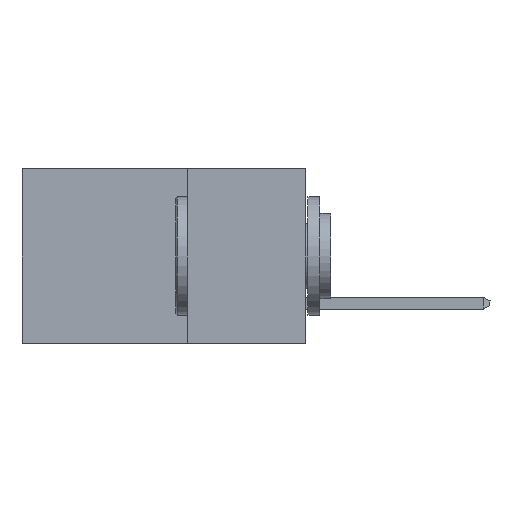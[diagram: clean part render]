
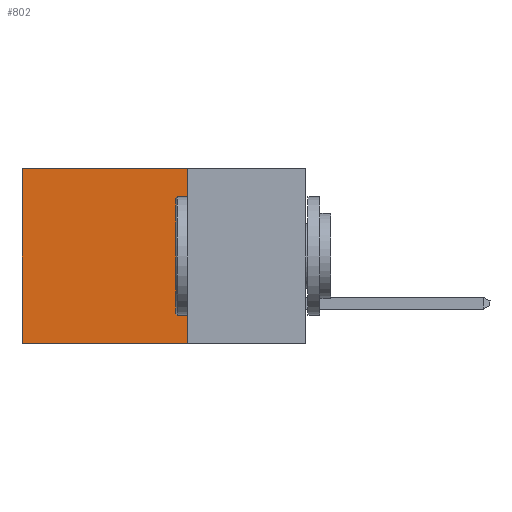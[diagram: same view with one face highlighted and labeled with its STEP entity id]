
A CAD part, left-side view. The second image highlights one B-rep face of the part: STEP entity #802.
In plain terms, the highlighted planar face has unit normal (-1, 0, 0).
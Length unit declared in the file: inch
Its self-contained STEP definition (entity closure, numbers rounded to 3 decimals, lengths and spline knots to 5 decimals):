
#802 = ADVANCED_FACE ( 'NONE', ( #961 ), #25187, .F. ) ;
#961 = FACE_OUTER_BOUND ( 'NONE', #20136, .T. ) ;
#1152 = DIRECTION ( 'NONE',  ( 0., 0., -1. ) ) ;
#1540 = ORIENTED_EDGE ( 'NONE', *, *, #11799, .F. ) ;
#1721 = CARTESIAN_POINT ( 'NONE',  ( 0.2615, 0.25, -0.37 ) ) ;
#3318 = AXIS2_PLACEMENT_3D ( 'NONE', #3454, #17326, #16933 ) ;
#3454 = CARTESIAN_POINT ( 'NONE',  ( 0.2615, 0.25, -0.37 ) ) ;
#3674 = CARTESIAN_POINT ( 'NONE',  ( 0.2615, 0.6, 0. ) ) ;
#5263 = ORIENTED_EDGE ( 'NONE', *, *, #16797, .T. ) ;
#6864 = DIRECTION ( 'NONE',  ( 0., 0., -1. ) ) ;
#7436 = CARTESIAN_POINT ( 'NONE',  ( 0.2615, 0.6, -0.37 ) ) ;
#8824 = CARTESIAN_POINT ( 'NONE',  ( 0.2615, 0.25, -0.37 ) ) ;
#9340 = EDGE_CURVE ( 'NONE', #10395, #18531, #11896, .T. ) ;
#10395 = VERTEX_POINT ( 'NONE', #16774 ) ;
#11387 = DIRECTION ( 'NONE',  ( 0., 1., 0. ) ) ;
#11799 = EDGE_CURVE ( 'NONE', #13001, #10395, #22992, .T. ) ;
#11896 = LINE ( 'NONE', #1721, #15910 ) ;
#12499 = EDGE_CURVE ( 'NONE', #13001, #13484, #16328, .T. ) ;
#13001 = VERTEX_POINT ( 'NONE', #23258 ) ;
#13072 = VECTOR ( 'NONE', #20791, 39.37008 ) ;
#13484 = VERTEX_POINT ( 'NONE', #3674 ) ;
#15272 = LINE ( 'NONE', #7436, #17797 ) ;
#15910 = VECTOR ( 'NONE', #11387, 39.37008 ) ;
#15977 = VECTOR ( 'NONE', #6864, 39.37008 ) ;
#16328 = LINE ( 'NONE', #18561, #13072 ) ;
#16774 = CARTESIAN_POINT ( 'NONE',  ( 0.2615, 0.25, -0.37 ) ) ;
#16797 = EDGE_CURVE ( 'NONE', #13484, #18531, #15272, .T. ) ;
#16933 = DIRECTION ( 'NONE',  ( 0., 0., -1. ) ) ;
#17326 = DIRECTION ( 'NONE',  ( 1., 0., 0. ) ) ;
#17409 = ORIENTED_EDGE ( 'NONE', *, *, #12499, .T. ) ;
#17797 = VECTOR ( 'NONE', #1152, 39.37008 ) ;
#18531 = VERTEX_POINT ( 'NONE', #22650 ) ;
#18561 = CARTESIAN_POINT ( 'NONE',  ( 0.2615, 0.25, 0. ) ) ;
#20136 = EDGE_LOOP ( 'NONE', ( #5263, #24698, #1540, #17409 ) ) ;
#20791 = DIRECTION ( 'NONE',  ( 0., 1., 0. ) ) ;
#22650 = CARTESIAN_POINT ( 'NONE',  ( 0.2615, 0.6, -0.37 ) ) ;
#22992 = LINE ( 'NONE', #8824, #15977 ) ;
#23258 = CARTESIAN_POINT ( 'NONE',  ( 0.2615, 0.25, 0. ) ) ;
#24698 = ORIENTED_EDGE ( 'NONE', *, *, #9340, .F. ) ;
#25187 = PLANE ( 'NONE',  #3318 ) ;
